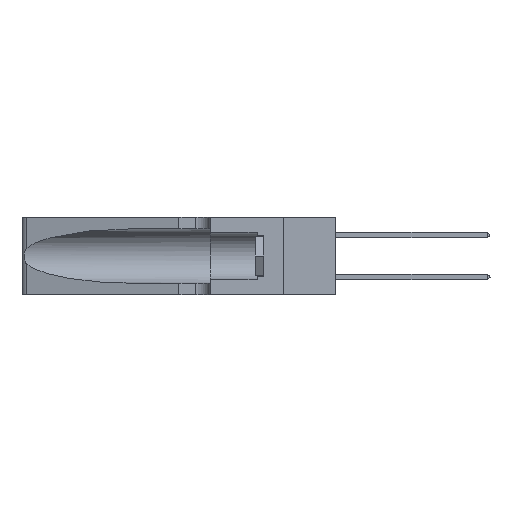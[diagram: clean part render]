
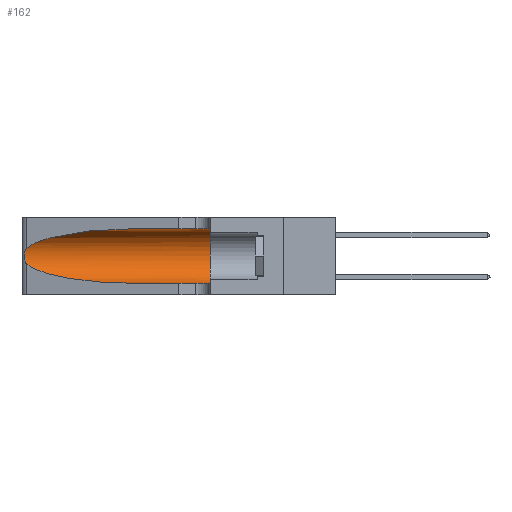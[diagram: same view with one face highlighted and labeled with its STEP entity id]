
A CAD part, left-side view. The second image highlights one B-rep face of the part: STEP entity #162.
In plain terms, the highlighted cylindrical face has radius 3.308 mm (diameter 6.617 mm), a partial arc.
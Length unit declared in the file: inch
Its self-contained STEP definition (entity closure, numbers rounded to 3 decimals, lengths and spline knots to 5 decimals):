
#162 = ADVANCED_FACE ( 'NONE', ( #5465 ), #8334, .F. ) ;
#370 = CARTESIAN_POINT ( 'NONE',  ( 0.1305, 0.35, 0.31525 ) ) ;
#751 = ORIENTED_EDGE ( 'NONE', *, *, #26008, .T. ) ;
#767 = DIRECTION ( 'NONE',  ( 0., -1., 0. ) ) ;
#2722 = CARTESIAN_POINT ( 'NONE',  ( 0.25787, 1.23484, 0.2124 ) ) ;
#3018 = CARTESIAN_POINT ( 'NONE',  ( 0.1305, 0.72297, 0.31525 ) ) ;
#3202 = CARTESIAN_POINT ( 'NONE',  ( 0.25555, 1.22993, 0.14849 ) ) ;
#3209 = CARTESIAN_POINT ( 'NONE',  ( 0.25487, 1.22718, 0.22369 ) ) ;
#3371 = ORIENTED_EDGE ( 'NONE', *, *, #5376, .T. ) ;
#4194 = CARTESIAN_POINT ( 'NONE',  ( 0.25487, 1.22718, 0.14631 ) ) ;
#4255 = CARTESIAN_POINT ( 'NONE',  ( 0.1305, 1.61858, 0.05475 ) ) ;
#4319 = EDGE_CURVE ( 'NONE', #13319, #29107, #23439, .T. ) ;
#4549 = EDGE_LOOP ( 'NONE', ( #751, #3371, #28333, #18512, #10948, #8161 ) ) ;
#4784 = CARTESIAN_POINT ( 'NONE',  ( 0.2373, 1.15595, 0.08982 ) ) ;
#5376 = EDGE_CURVE ( 'NONE', #27018, #29273, #10092, .T. ) ;
#5417 = VECTOR ( 'NONE', #5510, 39.37008 ) ;
#5465 = FACE_OUTER_BOUND ( 'NONE', #4549, .T. ) ;
#5510 = DIRECTION ( 'NONE',  ( 0., -1., 0. ) ) ;
#8161 = ORIENTED_EDGE ( 'NONE', *, *, #23591, .F. ) ;
#8334 = CYLINDRICAL_SURFACE ( 'NONE', #24967, 0.13025 ) ;
#8381 = CARTESIAN_POINT ( 'NONE',  ( 0.1305, 1.61858, 0.185 ) ) ;
#8482 = DIRECTION ( 'NONE',  ( 0., 0., 1. ) ) ;
#9250 = CARTESIAN_POINT ( 'NONE',  ( 0.1305, 0.72297, 0.05475 ) ) ;
#10092 = B_SPLINE_CURVE_WITH_KNOTS ( 'NONE', 3,
 ( #31658, #15635, #13123, #2722, #21573, #24029, #32056, #13681, #21455, #14273, #30077, #32415, #3202, #4194 ),
 .UNSPECIFIED., .F., .F.,
 ( 4, 2, 2, 2, 2, 2, 4 ),
 ( 0., 0.00027, 0.00053, 0.00107, 0.0016, 0.00187, 0.00214 ),
 .UNSPECIFIED. ) ;
#10948 = ORIENTED_EDGE ( 'NONE', *, *, #4319, .F. ) ;
#11389 =( BOUNDED_CURVE ( )  B_SPLINE_CURVE ( 3, ( #31065, #4784, #18015, #23150 ),
 .UNSPECIFIED., .F., .F. ) 
 B_SPLINE_CURVE_WITH_KNOTS ( ( 4, 4 ),
 ( 3.44316, 4.71239 ),
 .UNSPECIFIED. ) 
 CURVE ( )  GEOMETRIC_REPRESENTATION_ITEM ( )  RATIONAL_B_SPLINE_CURVE ( ( 1., 0.87, 0.87, 1. ) ) 
 REPRESENTATION_ITEM ( '' )  );
#12466 = VECTOR ( 'NONE', #17719, 39.37008 ) ;
#12925 = LINE ( 'NONE', #4255, #12466 ) ;
#13123 = CARTESIAN_POINT ( 'NONE',  ( 0.25639, 1.23184, 0.21858 ) ) ;
#13319 = VERTEX_POINT ( 'NONE', #370 ) ;
#13629 = CARTESIAN_POINT ( 'NONE',  ( 0.25487, 1.22718, 0.22369 ) ) ;
#13681 = CARTESIAN_POINT ( 'NONE',  ( 0.26075, 1.23896, 0.178 ) ) ;
#14074 = VERTEX_POINT ( 'NONE', #9250 ) ;
#14273 = CARTESIAN_POINT ( 'NONE',  ( 0.25856, 1.23593, 0.16098 ) ) ;
#15635 = CARTESIAN_POINT ( 'NONE',  ( 0.25555, 1.22994, 0.2215 ) ) ;
#16028 = CARTESIAN_POINT ( 'NONE',  ( 0.1305, 0.35, 0.185 ) ) ;
#16530 = EDGE_CURVE ( 'NONE', #29273, #14074, #11389, .T. ) ;
#17354 = CARTESIAN_POINT ( 'NONE',  ( 0.1305, 0.35, 0.05475 ) ) ;
#17719 = DIRECTION ( 'NONE',  ( 0., -1., 0. ) ) ;
#18015 = CARTESIAN_POINT ( 'NONE',  ( 0.18966, 0.96281, 0.05475 ) ) ;
#18074 = AXIS2_PLACEMENT_3D ( 'NONE', #16028, #24159, #8482 ) ;
#18512 = ORIENTED_EDGE ( 'NONE', *, *, #28630, .T. ) ;
#18968 = DIRECTION ( 'NONE',  ( 0., 0., -1. ) ) ;
#20380 = LINE ( 'NONE', #24459, #5417 ) ;
#21455 = CARTESIAN_POINT ( 'NONE',  ( 0.26017, 1.23833, 0.17102 ) ) ;
#21573 = CARTESIAN_POINT ( 'NONE',  ( 0.25854, 1.2359, 0.20912 ) ) ;
#21742 = CARTESIAN_POINT ( 'NONE',  ( 0.18966, 0.96281, 0.31525 ) ) ;
#22648 =( BOUNDED_CURVE ( )  B_SPLINE_CURVE ( 3, ( #3018, #21742, #29896, #13629 ),
 .UNSPECIFIED., .F., .F. ) 
 B_SPLINE_CURVE_WITH_KNOTS ( ( 4, 4 ),
 ( 1.5708, 2.84003 ),
 .UNSPECIFIED. ) 
 CURVE ( )  GEOMETRIC_REPRESENTATION_ITEM ( )  RATIONAL_B_SPLINE_CURVE ( ( 1., 0.87, 0.87, 1. ) ) 
 REPRESENTATION_ITEM ( '' )  );
#23150 = CARTESIAN_POINT ( 'NONE',  ( 0.1305, 0.72297, 0.05475 ) ) ;
#23439 = CIRCLE ( 'NONE', #18074, 0.13025 ) ;
#23591 = EDGE_CURVE ( 'NONE', #28568, #13319, #20380, .T. ) ;
#24029 = CARTESIAN_POINT ( 'NONE',  ( 0.26018, 1.23835, 0.19895 ) ) ;
#24159 = DIRECTION ( 'NONE',  ( 0., 1., 0. ) ) ;
#24459 = CARTESIAN_POINT ( 'NONE',  ( 0.1305, 1.61858, 0.31525 ) ) ;
#24967 = AXIS2_PLACEMENT_3D ( 'NONE', #8381, #767, #18968 ) ;
#26008 = EDGE_CURVE ( 'NONE', #28568, #27018, #22648, .T. ) ;
#26417 = CARTESIAN_POINT ( 'NONE',  ( 0.25487, 1.22718, 0.14631 ) ) ;
#27018 = VERTEX_POINT ( 'NONE', #3209 ) ;
#28333 = ORIENTED_EDGE ( 'NONE', *, *, #16530, .T. ) ;
#28568 = VERTEX_POINT ( 'NONE', #30331 ) ;
#28630 = EDGE_CURVE ( 'NONE', #14074, #29107, #12925, .T. ) ;
#29107 = VERTEX_POINT ( 'NONE', #17354 ) ;
#29273 = VERTEX_POINT ( 'NONE', #26417 ) ;
#29896 = CARTESIAN_POINT ( 'NONE',  ( 0.2373, 1.15595, 0.28018 ) ) ;
#30077 = CARTESIAN_POINT ( 'NONE',  ( 0.25789, 1.23486, 0.15765 ) ) ;
#30331 = CARTESIAN_POINT ( 'NONE',  ( 0.1305, 0.72297, 0.31525 ) ) ;
#31065 = CARTESIAN_POINT ( 'NONE',  ( 0.25487, 1.22718, 0.14631 ) ) ;
#31658 = CARTESIAN_POINT ( 'NONE',  ( 0.25487, 1.22718, 0.22369 ) ) ;
#32056 = CARTESIAN_POINT ( 'NONE',  ( 0.26075, 1.23896, 0.19203 ) ) ;
#32415 = CARTESIAN_POINT ( 'NONE',  ( 0.25639, 1.23186, 0.15144 ) ) ;
